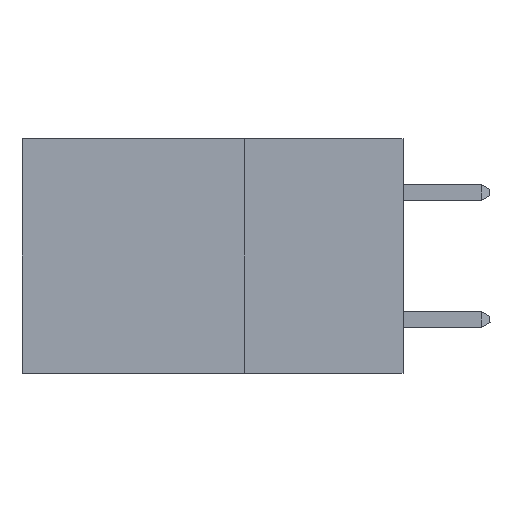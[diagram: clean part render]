
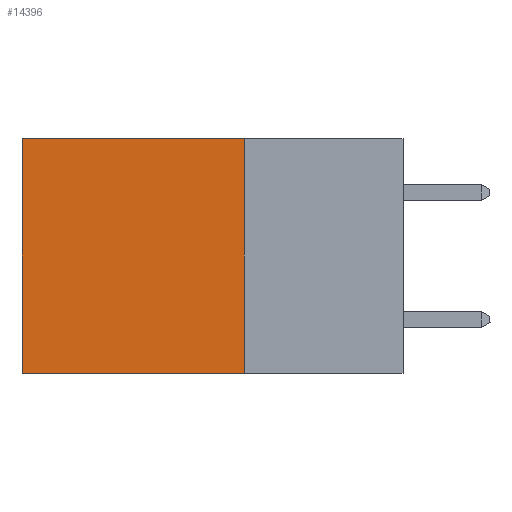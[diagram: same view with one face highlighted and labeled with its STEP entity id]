
A CAD part, left-side view. The second image highlights one B-rep face of the part: STEP entity #14396.
In plain terms, the highlighted planar face has unit normal (-1, 0, 0).
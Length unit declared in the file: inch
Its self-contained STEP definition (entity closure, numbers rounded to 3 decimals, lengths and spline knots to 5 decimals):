
#2464 = VERTEX_POINT ( 'NONE', #14585 ) ;
#3315 = DIRECTION ( 'NONE',  ( 1., 0., 0. ) ) ;
#3519 = CARTESIAN_POINT ( 'NONE',  ( 0.2875, 0.25, 0. ) ) ;
#3679 = CARTESIAN_POINT ( 'NONE',  ( 0.2875, 0.25, -0.37 ) ) ;
#4190 = VERTEX_POINT ( 'NONE', #21856 ) ;
#7069 = VECTOR ( 'NONE', #9469, 39.37008 ) ;
#8270 = EDGE_LOOP ( 'NONE', ( #30370, #22373, #25985, #28328 ) ) ;
#9370 = CARTESIAN_POINT ( 'NONE',  ( 0.2875, 0.25, 0. ) ) ;
#9469 = DIRECTION ( 'NONE',  ( 0., 0., -1. ) ) ;
#9558 = EDGE_CURVE ( 'NONE', #13318, #2464, #23827, .T. ) ;
#9973 = AXIS2_PLACEMENT_3D ( 'NONE', #3519, #3315, #27125 ) ;
#10774 = EDGE_CURVE ( 'NONE', #27428, #2464, #25970, .T. ) ;
#10979 = CARTESIAN_POINT ( 'NONE',  ( 0.2875, 0.25, 0. ) ) ;
#13318 = VERTEX_POINT ( 'NONE', #24121 ) ;
#13343 = LINE ( 'NONE', #9370, #7069 ) ;
#13475 = LINE ( 'NONE', #10979, #20526 ) ;
#14396 = ADVANCED_FACE ( 'NONE', ( #21893 ), #17404, .F. ) ;
#14585 = CARTESIAN_POINT ( 'NONE',  ( 0.2875, 0.6, -0.37 ) ) ;
#17404 = PLANE ( 'NONE',  #9973 ) ;
#17922 = EDGE_CURVE ( 'NONE', #4190, #13318, #13475, .T. ) ;
#20526 = VECTOR ( 'NONE', #27273, 39.37008 ) ;
#20565 = VECTOR ( 'NONE', #22695, 39.37008 ) ;
#21856 = CARTESIAN_POINT ( 'NONE',  ( 0.2875, 0.25, 0. ) ) ;
#21893 = FACE_OUTER_BOUND ( 'NONE', #8270, .T. ) ;
#22373 = ORIENTED_EDGE ( 'NONE', *, *, #10774, .F. ) ;
#22695 = DIRECTION ( 'NONE',  ( 0., 0., -1. ) ) ;
#23827 = LINE ( 'NONE', #24436, #20565 ) ;
#24121 = CARTESIAN_POINT ( 'NONE',  ( 0.2875, 0.6, 0. ) ) ;
#24436 = CARTESIAN_POINT ( 'NONE',  ( 0.2875, 0.6, 0. ) ) ;
#25970 = LINE ( 'NONE', #29660, #26694 ) ;
#25985 = ORIENTED_EDGE ( 'NONE', *, *, #29240, .F. ) ;
#26694 = VECTOR ( 'NONE', #29771, 39.37008 ) ;
#27125 = DIRECTION ( 'NONE',  ( 0., 0., -1. ) ) ;
#27273 = DIRECTION ( 'NONE',  ( 0., 1., 0. ) ) ;
#27428 = VERTEX_POINT ( 'NONE', #3679 ) ;
#28328 = ORIENTED_EDGE ( 'NONE', *, *, #17922, .T. ) ;
#29240 = EDGE_CURVE ( 'NONE', #4190, #27428, #13343, .T. ) ;
#29660 = CARTESIAN_POINT ( 'NONE',  ( 0.2875, 0.25, -0.37 ) ) ;
#29771 = DIRECTION ( 'NONE',  ( 0., 1., 0. ) ) ;
#30370 = ORIENTED_EDGE ( 'NONE', *, *, #9558, .T. ) ;
